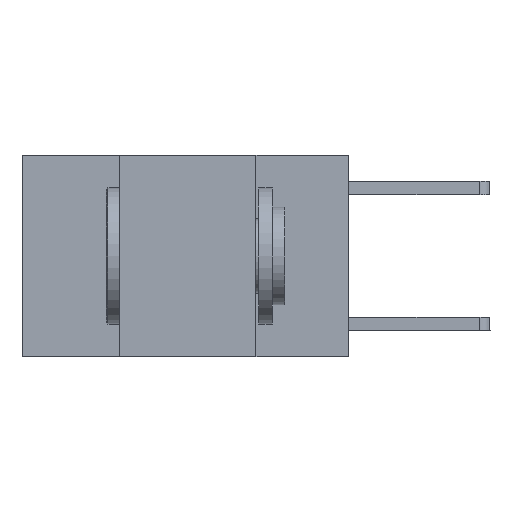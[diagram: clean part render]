
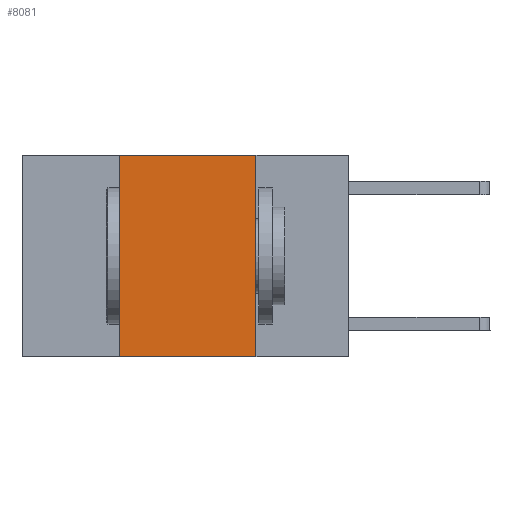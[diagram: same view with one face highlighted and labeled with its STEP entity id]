
A CAD part, left-side view. The second image highlights one B-rep face of the part: STEP entity #8081.
In plain terms, the highlighted planar face has unit normal (-1, 0, 0).
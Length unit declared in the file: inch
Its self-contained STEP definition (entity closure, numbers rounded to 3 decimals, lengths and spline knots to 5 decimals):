
#271 = ORIENTED_EDGE ( 'NONE', *, *, #5166, .F. ) ;
#403 = VERTEX_POINT ( 'NONE', #3772 ) ;
#537 = ORIENTED_EDGE ( 'NONE', *, *, #4110, .F. ) ;
#764 = LINE ( 'NONE', #3736, #4922 ) ;
#1562 = LINE ( 'NONE', #8748, #7850 ) ;
#1652 = CARTESIAN_POINT ( 'NONE',  ( 0., 0.17, -0.37 ) ) ;
#1742 = CARTESIAN_POINT ( 'NONE',  ( 0., 0.42, 0. ) ) ;
#1855 = PLANE ( 'NONE',  #3620 ) ;
#2841 = DIRECTION ( 'NONE',  ( 0., 0., 1. ) ) ;
#2911 = VERTEX_POINT ( 'NONE', #4493 ) ;
#3377 = EDGE_LOOP ( 'NONE', ( #10190, #537, #271, #10271 ) ) ;
#3392 = VERTEX_POINT ( 'NONE', #1652 ) ;
#3463 = LINE ( 'NONE', #3676, #9594 ) ;
#3478 = DIRECTION ( 'NONE',  ( 1., 0., 0. ) ) ;
#3620 = AXIS2_PLACEMENT_3D ( 'NONE', #4274, #3478, #9105 ) ;
#3638 = DIRECTION ( 'NONE',  ( 0., 0., -1. ) ) ;
#3676 = CARTESIAN_POINT ( 'NONE',  ( 0., 0.42, 0. ) ) ;
#3736 = CARTESIAN_POINT ( 'NONE',  ( 0., 0.6, -0.37 ) ) ;
#3772 = CARTESIAN_POINT ( 'NONE',  ( 0., 0.17, 0. ) ) ;
#3903 = DIRECTION ( 'NONE',  ( 0., -1., 0. ) ) ;
#4110 = EDGE_CURVE ( 'NONE', #5990, #403, #1562, .T. ) ;
#4274 = CARTESIAN_POINT ( 'NONE',  ( 0., 0.6, 0. ) ) ;
#4493 = CARTESIAN_POINT ( 'NONE',  ( 0., 0.42, -0.37 ) ) ;
#4597 = DIRECTION ( 'NONE',  ( 0., -1., 0. ) ) ;
#4922 = VECTOR ( 'NONE', #4597, 39.37008 ) ;
#5152 = EDGE_CURVE ( 'NONE', #403, #3392, #7857, .T. ) ;
#5166 = EDGE_CURVE ( 'NONE', #2911, #5990, #3463, .T. ) ;
#5200 = EDGE_CURVE ( 'NONE', #2911, #3392, #764, .T. ) ;
#5907 = FACE_OUTER_BOUND ( 'NONE', #3377, .T. ) ;
#5990 = VERTEX_POINT ( 'NONE', #1742 ) ;
#6190 = CARTESIAN_POINT ( 'NONE',  ( 0., 0.17, 0. ) ) ;
#7850 = VECTOR ( 'NONE', #3903, 39.37008 ) ;
#7857 = LINE ( 'NONE', #6190, #9824 ) ;
#8081 = ADVANCED_FACE ( 'NONE', ( #5907 ), #1855, .F. ) ;
#8748 = CARTESIAN_POINT ( 'NONE',  ( 0., 0.6, 0. ) ) ;
#9105 = DIRECTION ( 'NONE',  ( 0., 0., -1. ) ) ;
#9594 = VECTOR ( 'NONE', #2841, 39.37008 ) ;
#9824 = VECTOR ( 'NONE', #3638, 39.37008 ) ;
#10190 = ORIENTED_EDGE ( 'NONE', *, *, #5152, .F. ) ;
#10271 = ORIENTED_EDGE ( 'NONE', *, *, #5200, .T. ) ;
